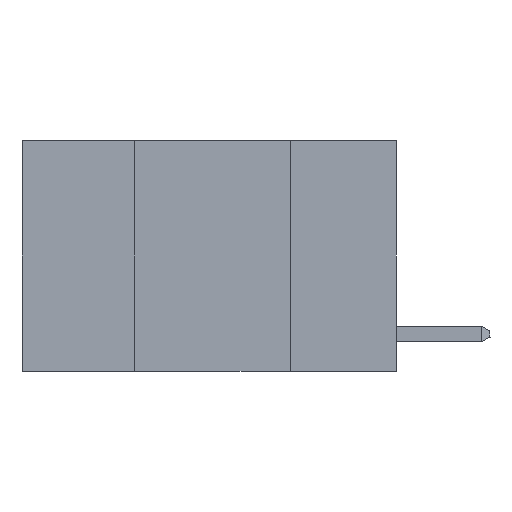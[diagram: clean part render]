
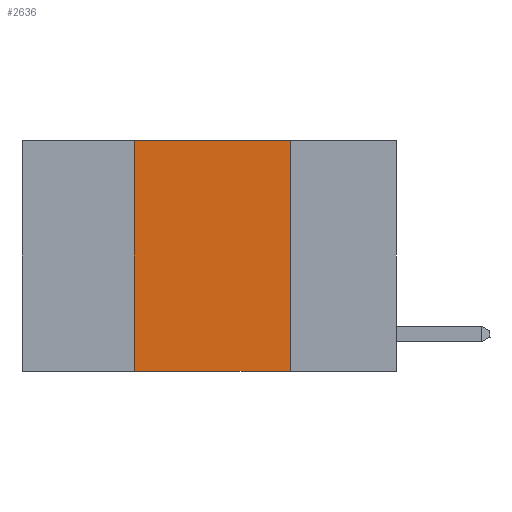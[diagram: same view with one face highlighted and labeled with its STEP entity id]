
A CAD part, left-side view. The second image highlights one B-rep face of the part: STEP entity #2636.
In plain terms, the highlighted planar face has unit normal (-1, 0, 0).
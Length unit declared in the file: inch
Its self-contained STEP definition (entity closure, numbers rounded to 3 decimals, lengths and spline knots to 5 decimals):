
#402 = CARTESIAN_POINT ( 'NONE',  ( 0., 0.17, 0. ) ) ;
#1355 = DIRECTION ( 'NONE',  ( 0., -1., 0. ) ) ;
#1536 = VERTEX_POINT ( 'NONE', #17467 ) ;
#2636 = ADVANCED_FACE ( 'NONE', ( #21266 ), #11372, .F. ) ;
#2717 = LINE ( 'NONE', #7781, #16920 ) ;
#4575 = CARTESIAN_POINT ( 'NONE',  ( 0., 0.42, -0.37 ) ) ;
#4592 = VECTOR ( 'NONE', #15893, 39.37008 ) ;
#5953 = VERTEX_POINT ( 'NONE', #20773 ) ;
#7781 = CARTESIAN_POINT ( 'NONE',  ( 0., 0.6, -0.37 ) ) ;
#8442 = CARTESIAN_POINT ( 'NONE',  ( 0., 0.42, 0. ) ) ;
#8898 = EDGE_CURVE ( 'NONE', #14118, #5953, #21060, .T. ) ;
#9168 = CARTESIAN_POINT ( 'NONE',  ( 0., 0.17, 0. ) ) ;
#9635 = CARTESIAN_POINT ( 'NONE',  ( 0., 0.6, 0. ) ) ;
#11150 = ORIENTED_EDGE ( 'NONE', *, *, #18915, .T. ) ;
#11372 = PLANE ( 'NONE',  #13659 ) ;
#11706 = EDGE_CURVE ( 'NONE', #1536, #14118, #16451, .T. ) ;
#12941 = VECTOR ( 'NONE', #20236, 39.37008 ) ;
#13536 = LINE ( 'NONE', #8442, #12941 ) ;
#13659 = AXIS2_PLACEMENT_3D ( 'NONE', #21359, #18087, #21599 ) ;
#13972 = EDGE_CURVE ( 'NONE', #17413, #1536, #13536, .T. ) ;
#14118 = VERTEX_POINT ( 'NONE', #402 ) ;
#14528 = DIRECTION ( 'NONE',  ( 0., -1., 0. ) ) ;
#15893 = DIRECTION ( 'NONE',  ( 0., 0., -1. ) ) ;
#15897 = VECTOR ( 'NONE', #1355, 39.37008 ) ;
#16451 = LINE ( 'NONE', #9635, #15897 ) ;
#16730 = ORIENTED_EDGE ( 'NONE', *, *, #11706, .F. ) ;
#16920 = VECTOR ( 'NONE', #14528, 39.37008 ) ;
#17413 = VERTEX_POINT ( 'NONE', #4575 ) ;
#17467 = CARTESIAN_POINT ( 'NONE',  ( 0., 0.42, 0. ) ) ;
#18087 = DIRECTION ( 'NONE',  ( 1., 0., 0. ) ) ;
#18915 = EDGE_CURVE ( 'NONE', #17413, #5953, #2717, .T. ) ;
#20171 = EDGE_LOOP ( 'NONE', ( #20802, #16730, #21105, #11150 ) ) ;
#20236 = DIRECTION ( 'NONE',  ( 0., 0., 1. ) ) ;
#20773 = CARTESIAN_POINT ( 'NONE',  ( 0., 0.17, -0.37 ) ) ;
#20802 = ORIENTED_EDGE ( 'NONE', *, *, #8898, .F. ) ;
#21060 = LINE ( 'NONE', #9168, #4592 ) ;
#21105 = ORIENTED_EDGE ( 'NONE', *, *, #13972, .F. ) ;
#21266 = FACE_OUTER_BOUND ( 'NONE', #20171, .T. ) ;
#21359 = CARTESIAN_POINT ( 'NONE',  ( 0., 0.6, 0. ) ) ;
#21599 = DIRECTION ( 'NONE',  ( 0., 0., -1. ) ) ;
